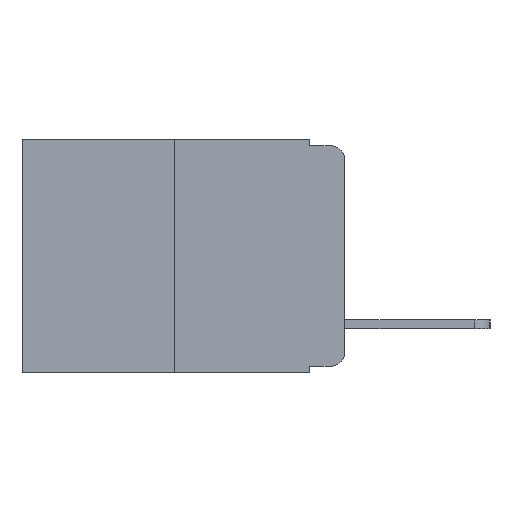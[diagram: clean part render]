
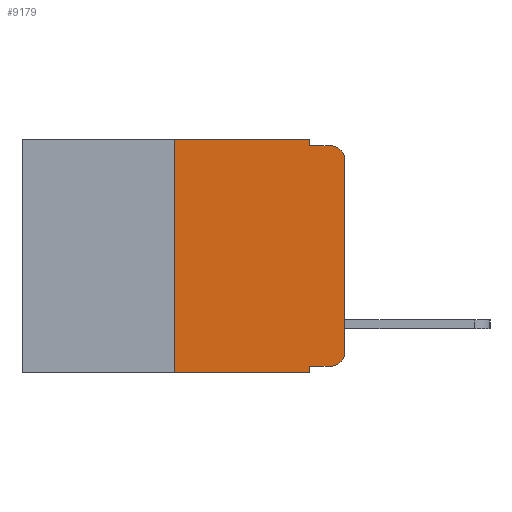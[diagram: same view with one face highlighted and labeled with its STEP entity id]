
A CAD part, left-side view. The second image highlights one B-rep face of the part: STEP entity #9179.
In plain terms, the highlighted planar face has unit normal (-1, 0, 0).
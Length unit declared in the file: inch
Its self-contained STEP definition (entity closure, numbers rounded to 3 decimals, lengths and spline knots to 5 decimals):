
#503 = CARTESIAN_POINT ( 'NONE',  ( 0., 0.051, 0. ) ) ;
#541 = AXIS2_PLACEMENT_3D ( 'NONE', #21944, #23772, #12692 ) ;
#833 = LINE ( 'NONE', #23153, #6035 ) ;
#847 = CIRCLE ( 'NONE', #19078, 0.02 ) ;
#940 = EDGE_CURVE ( 'NONE', #17959, #6412, #3628, .T. ) ;
#1264 = EDGE_CURVE ( 'NONE', #13498, #5537, #833, .T. ) ;
#1365 = LINE ( 'NONE', #16070, #5981 ) ;
#1528 = ORIENTED_EDGE ( 'NONE', *, *, #24152, .F. ) ;
#2333 = CARTESIAN_POINT ( 'NONE',  ( 0., 0.051, 0. ) ) ;
#2473 = DIRECTION ( 'NONE',  ( 0., 0., -1. ) ) ;
#3628 = LINE ( 'NONE', #11994, #22445 ) ;
#3928 = AXIS2_PLACEMENT_3D ( 'NONE', #7792, #20838, #9683 ) ;
#4520 = LINE ( 'NONE', #10721, #14008 ) ;
#4661 = ORIENTED_EDGE ( 'NONE', *, *, #4892, .T. ) ;
#4715 = LINE ( 'NONE', #503, #14192 ) ;
#4767 = CARTESIAN_POINT ( 'NONE',  ( 0., 0.051, 0. ) ) ;
#4799 = CARTESIAN_POINT ( 'NONE',  ( 0., 0.051, -0.333 ) ) ;
#4892 = EDGE_CURVE ( 'NONE', #14092, #6412, #847, .T. ) ;
#5140 = VERTEX_POINT ( 'NONE', #14910 ) ;
#5537 = VERTEX_POINT ( 'NONE', #6584 ) ;
#5881 = ORIENTED_EDGE ( 'NONE', *, *, #940, .F. ) ;
#5981 = VECTOR ( 'NONE', #8646, 39.37008 ) ;
#6035 = VECTOR ( 'NONE', #24237, 39.37008 ) ;
#6197 = EDGE_CURVE ( 'NONE', #13861, #14092, #1365, .T. ) ;
#6412 = VERTEX_POINT ( 'NONE', #14772 ) ;
#6446 = DIRECTION ( 'NONE',  ( -1., 0., 0. ) ) ;
#6465 = CARTESIAN_POINT ( 'NONE',  ( 0., 0., -0.313 ) ) ;
#6541 = CARTESIAN_POINT ( 'NONE',  ( 0., 0.051, -0.333 ) ) ;
#6584 = CARTESIAN_POINT ( 'NONE',  ( 0., 0.051, -0.343 ) ) ;
#6716 = DIRECTION ( 'NONE',  ( 0., 0., -1. ) ) ;
#6740 = ORIENTED_EDGE ( 'NONE', *, *, #20640, .F. ) ;
#6887 = CARTESIAN_POINT ( 'NONE',  ( 0., 0.02, -0.333 ) ) ;
#7354 = ORIENTED_EDGE ( 'NONE', *, *, #20455, .F. ) ;
#7792 = CARTESIAN_POINT ( 'NONE',  ( 0., 0.02, -0.313 ) ) ;
#8464 = DIRECTION ( 'NONE',  ( 0., -1., 0. ) ) ;
#8573 = ORIENTED_EDGE ( 'NONE', *, *, #6197, .T. ) ;
#8646 = DIRECTION ( 'NONE',  ( 0., 0., 1. ) ) ;
#9179 = ADVANCED_FACE ( 'NONE', ( #9752 ), #20054, .F. ) ;
#9683 = DIRECTION ( 'NONE',  ( 0., 0., -1. ) ) ;
#9752 = FACE_OUTER_BOUND ( 'NONE', #12274, .T. ) ;
#10721 = CARTESIAN_POINT ( 'NONE',  ( 0., 0.25, 0. ) ) ;
#10741 = LINE ( 'NONE', #6541, #15127 ) ;
#11066 = LINE ( 'NONE', #20554, #19796 ) ;
#11994 = CARTESIAN_POINT ( 'NONE',  ( 0., 0.051, -0.01 ) ) ;
#12178 = VERTEX_POINT ( 'NONE', #2333 ) ;
#12274 = EDGE_LOOP ( 'NONE', ( #8573, #4661, #5881, #1528, #6740, #7354, #17297, #22236, #23397, #20191 ) ) ;
#12337 = VERTEX_POINT ( 'NONE', #4799 ) ;
#12617 = DIRECTION ( 'NONE',  ( 0., 0., 1. ) ) ;
#12692 = DIRECTION ( 'NONE',  ( 0., 0., -1. ) ) ;
#12904 = VECTOR ( 'NONE', #6716, 39.37008 ) ;
#13491 = LINE ( 'NONE', #4767, #12904 ) ;
#13498 = VERTEX_POINT ( 'NONE', #24003 ) ;
#13861 = VERTEX_POINT ( 'NONE', #6465 ) ;
#14008 = VECTOR ( 'NONE', #12617, 39.37008 ) ;
#14092 = VERTEX_POINT ( 'NONE', #22132 ) ;
#14192 = VECTOR ( 'NONE', #2473, 39.37008 ) ;
#14243 = EDGE_CURVE ( 'NONE', #22480, #13861, #18991, .T. ) ;
#14772 = CARTESIAN_POINT ( 'NONE',  ( 0., 0.02, -0.01 ) ) ;
#14910 = CARTESIAN_POINT ( 'NONE',  ( 0., 0.25, 0. ) ) ;
#15127 = VECTOR ( 'NONE', #8464, 39.37008 ) ;
#16070 = CARTESIAN_POINT ( 'NONE',  ( 0., 0., 0. ) ) ;
#17297 = ORIENTED_EDGE ( 'NONE', *, *, #1264, .T. ) ;
#17444 = DIRECTION ( 'NONE',  ( 0., -1., 0. ) ) ;
#17672 = CARTESIAN_POINT ( 'NONE',  ( 0., 0.02, -0.03 ) ) ;
#17959 = VERTEX_POINT ( 'NONE', #21445 ) ;
#17973 = EDGE_CURVE ( 'NONE', #12337, #22480, #10741, .T. ) ;
#18991 = CIRCLE ( 'NONE', #3928, 0.02 ) ;
#19078 = AXIS2_PLACEMENT_3D ( 'NONE', #17672, #6446, #19538 ) ;
#19217 = EDGE_CURVE ( 'NONE', #12337, #5537, #13491, .T. ) ;
#19538 = DIRECTION ( 'NONE',  ( 0., 0., -1. ) ) ;
#19796 = VECTOR ( 'NONE', #22418, 39.37008 ) ;
#20054 = PLANE ( 'NONE',  #541 ) ;
#20191 = ORIENTED_EDGE ( 'NONE', *, *, #14243, .T. ) ;
#20455 = EDGE_CURVE ( 'NONE', #13498, #5140, #4520, .T. ) ;
#20554 = CARTESIAN_POINT ( 'NONE',  ( 0., 0.473, 0. ) ) ;
#20640 = EDGE_CURVE ( 'NONE', #5140, #12178, #11066, .T. ) ;
#20838 = DIRECTION ( 'NONE',  ( -1., 0., 0. ) ) ;
#21445 = CARTESIAN_POINT ( 'NONE',  ( 0., 0.051, -0.01 ) ) ;
#21944 = CARTESIAN_POINT ( 'NONE',  ( 0., 0.473, 0. ) ) ;
#22132 = CARTESIAN_POINT ( 'NONE',  ( 0., 0., -0.03 ) ) ;
#22236 = ORIENTED_EDGE ( 'NONE', *, *, #19217, .F. ) ;
#22418 = DIRECTION ( 'NONE',  ( 0., -1., 0. ) ) ;
#22445 = VECTOR ( 'NONE', #17444, 39.37008 ) ;
#22480 = VERTEX_POINT ( 'NONE', #6887 ) ;
#23153 = CARTESIAN_POINT ( 'NONE',  ( 0., 0.473, -0.343 ) ) ;
#23397 = ORIENTED_EDGE ( 'NONE', *, *, #17973, .T. ) ;
#23772 = DIRECTION ( 'NONE',  ( 1., 0., 0. ) ) ;
#24003 = CARTESIAN_POINT ( 'NONE',  ( 0., 0.25, -0.343 ) ) ;
#24152 = EDGE_CURVE ( 'NONE', #12178, #17959, #4715, .T. ) ;
#24237 = DIRECTION ( 'NONE',  ( 0., -1., 0. ) ) ;
